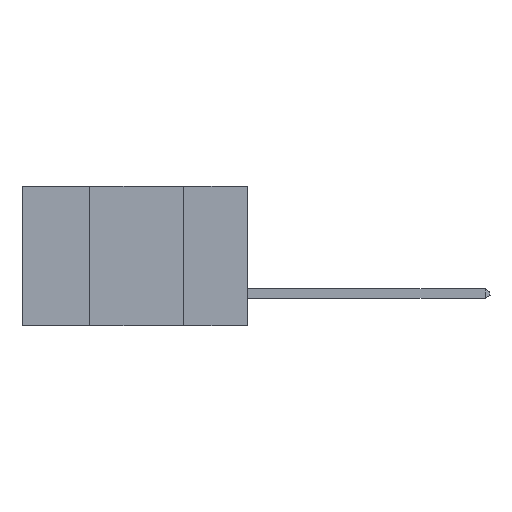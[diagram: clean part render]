
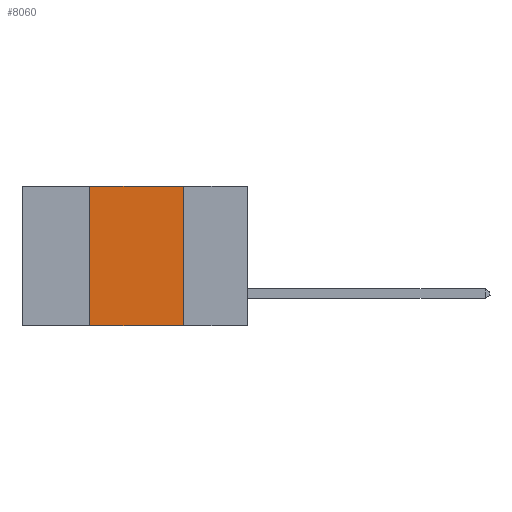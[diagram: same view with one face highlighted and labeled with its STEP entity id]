
A CAD part, left-side view. The second image highlights one B-rep face of the part: STEP entity #8060.
In plain terms, the highlighted planar face has unit normal (-1, 0, 0).
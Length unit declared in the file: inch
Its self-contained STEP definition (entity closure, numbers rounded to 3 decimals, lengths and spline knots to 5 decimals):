
#626 = CARTESIAN_POINT ( 'NONE',  ( 0., 0.17, 0. ) ) ;
#673 = VECTOR ( 'NONE', #6562, 39.37008 ) ;
#1220 = LINE ( 'NONE', #6507, #7768 ) ;
#1580 = VERTEX_POINT ( 'NONE', #8386 ) ;
#1659 = VECTOR ( 'NONE', #6221, 39.37008 ) ;
#1867 = DIRECTION ( 'NONE',  ( 1., 0., 0. ) ) ;
#2247 = EDGE_LOOP ( 'NONE', ( #8894, #8969, #4630, #5534 ) ) ;
#3751 = VERTEX_POINT ( 'NONE', #9933 ) ;
#4628 = CARTESIAN_POINT ( 'NONE',  ( 0., 0.17, 0. ) ) ;
#4630 = ORIENTED_EDGE ( 'NONE', *, *, #8797, .F. ) ;
#4643 = FACE_OUTER_BOUND ( 'NONE', #2247, .T. ) ;
#5262 = CARTESIAN_POINT ( 'NONE',  ( 0., 0.6, 0. ) ) ;
#5534 = ORIENTED_EDGE ( 'NONE', *, *, #7468, .T. ) ;
#5918 = VERTEX_POINT ( 'NONE', #4628 ) ;
#6221 = DIRECTION ( 'NONE',  ( 0., 0., 1. ) ) ;
#6507 = CARTESIAN_POINT ( 'NONE',  ( 0., 0.6, 0. ) ) ;
#6562 = DIRECTION ( 'NONE',  ( 0., 0., -1. ) ) ;
#6822 = LINE ( 'NONE', #626, #673 ) ;
#7468 = EDGE_CURVE ( 'NONE', #1580, #3751, #10561, .T. ) ;
#7485 = CARTESIAN_POINT ( 'NONE',  ( 0., 0.42, 0. ) ) ;
#7768 = VECTOR ( 'NONE', #9980, 39.37008 ) ;
#7952 = DIRECTION ( 'NONE',  ( 0., -1., 0. ) ) ;
#8004 = VERTEX_POINT ( 'NONE', #7485 ) ;
#8060 = ADVANCED_FACE ( 'NONE', ( #4643 ), #10353, .F. ) ;
#8332 = LINE ( 'NONE', #9682, #1659 ) ;
#8386 = CARTESIAN_POINT ( 'NONE',  ( 0., 0.42, -0.37 ) ) ;
#8797 = EDGE_CURVE ( 'NONE', #1580, #8004, #8332, .T. ) ;
#8894 = ORIENTED_EDGE ( 'NONE', *, *, #10706, .F. ) ;
#8969 = ORIENTED_EDGE ( 'NONE', *, *, #10102, .F. ) ;
#9493 = DIRECTION ( 'NONE',  ( 0., 0., -1. ) ) ;
#9606 = CARTESIAN_POINT ( 'NONE',  ( 0., 0.6, -0.37 ) ) ;
#9682 = CARTESIAN_POINT ( 'NONE',  ( 0., 0.42, 0. ) ) ;
#9933 = CARTESIAN_POINT ( 'NONE',  ( 0., 0.17, -0.37 ) ) ;
#9980 = DIRECTION ( 'NONE',  ( 0., -1., 0. ) ) ;
#10102 = EDGE_CURVE ( 'NONE', #8004, #5918, #1220, .T. ) ;
#10353 = PLANE ( 'NONE',  #10540 ) ;
#10540 = AXIS2_PLACEMENT_3D ( 'NONE', #5262, #1867, #9493 ) ;
#10561 = LINE ( 'NONE', #9606, #10815 ) ;
#10706 = EDGE_CURVE ( 'NONE', #5918, #3751, #6822, .T. ) ;
#10815 = VECTOR ( 'NONE', #7952, 39.37008 ) ;
